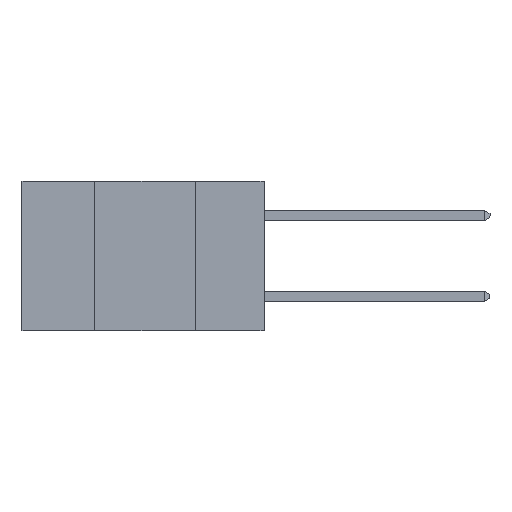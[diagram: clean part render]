
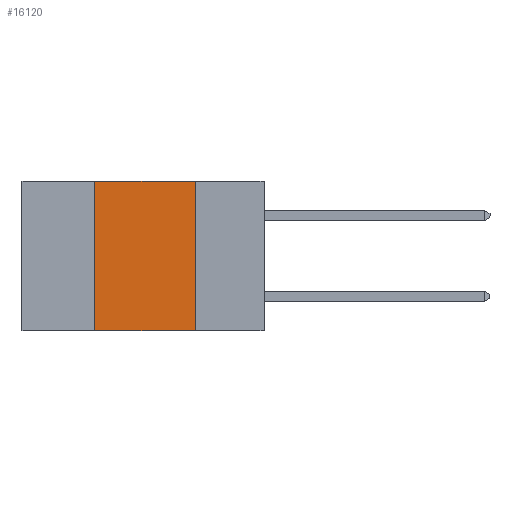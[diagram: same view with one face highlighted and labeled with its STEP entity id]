
A CAD part, left-side view. The second image highlights one B-rep face of the part: STEP entity #16120.
In plain terms, the highlighted planar face has unit normal (-1, 0, 0).
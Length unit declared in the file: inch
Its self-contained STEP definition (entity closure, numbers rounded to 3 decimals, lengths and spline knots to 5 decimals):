
#268 = LINE ( 'NONE', #8152, #11005 ) ;
#854 = VERTEX_POINT ( 'NONE', #11693 ) ;
#874 = VERTEX_POINT ( 'NONE', #18136 ) ;
#1328 = EDGE_CURVE ( 'NONE', #6821, #854, #14508, .T. ) ;
#3621 = DIRECTION ( 'NONE',  ( 0., -1., 0. ) ) ;
#4581 = ORIENTED_EDGE ( 'NONE', *, *, #21977, .F. ) ;
#5071 = DIRECTION ( 'NONE',  ( 1., 0., 0. ) ) ;
#6821 = VERTEX_POINT ( 'NONE', #22107 ) ;
#6825 = AXIS2_PLACEMENT_3D ( 'NONE', #12599, #5071, #18174 ) ;
#6891 = EDGE_LOOP ( 'NONE', ( #16045, #7476, #4581, #7815 ) ) ;
#7476 = ORIENTED_EDGE ( 'NONE', *, *, #23060, .F. ) ;
#7486 = DIRECTION ( 'NONE',  ( 0., -1., 0. ) ) ;
#7506 = DIRECTION ( 'NONE',  ( 0., 0., -1. ) ) ;
#7815 = ORIENTED_EDGE ( 'NONE', *, *, #20712, .T. ) ;
#8019 = CARTESIAN_POINT ( 'NONE',  ( 0., 0.17, 0. ) ) ;
#8152 = CARTESIAN_POINT ( 'NONE',  ( 0., 0.42, 0. ) ) ;
#8969 = LINE ( 'NONE', #14918, #13336 ) ;
#9570 = VECTOR ( 'NONE', #7506, 39.37008 ) ;
#11005 = VECTOR ( 'NONE', #21247, 39.37008 ) ;
#11105 = LINE ( 'NONE', #18573, #15458 ) ;
#11693 = CARTESIAN_POINT ( 'NONE',  ( 0., 0.17, -0.37 ) ) ;
#12599 = CARTESIAN_POINT ( 'NONE',  ( 0., 0.6, 0. ) ) ;
#13336 = VECTOR ( 'NONE', #7486, 39.37008 ) ;
#14508 = LINE ( 'NONE', #8019, #9570 ) ;
#14918 = CARTESIAN_POINT ( 'NONE',  ( 0., 0.6, -0.37 ) ) ;
#15458 = VECTOR ( 'NONE', #3621, 39.37008 ) ;
#15871 = CARTESIAN_POINT ( 'NONE',  ( 0., 0.42, -0.37 ) ) ;
#16045 = ORIENTED_EDGE ( 'NONE', *, *, #1328, .F. ) ;
#16120 = ADVANCED_FACE ( 'NONE', ( #23876 ), #18096, .F. ) ;
#18096 = PLANE ( 'NONE',  #6825 ) ;
#18136 = CARTESIAN_POINT ( 'NONE',  ( 0., 0.42, 0. ) ) ;
#18174 = DIRECTION ( 'NONE',  ( 0., 0., -1. ) ) ;
#18573 = CARTESIAN_POINT ( 'NONE',  ( 0., 0.6, 0. ) ) ;
#19818 = VERTEX_POINT ( 'NONE', #15871 ) ;
#20712 = EDGE_CURVE ( 'NONE', #19818, #854, #8969, .T. ) ;
#21247 = DIRECTION ( 'NONE',  ( 0., 0., 1. ) ) ;
#21977 = EDGE_CURVE ( 'NONE', #19818, #874, #268, .T. ) ;
#22107 = CARTESIAN_POINT ( 'NONE',  ( 0., 0.17, 0. ) ) ;
#23060 = EDGE_CURVE ( 'NONE', #874, #6821, #11105, .T. ) ;
#23876 = FACE_OUTER_BOUND ( 'NONE', #6891, .T. ) ;
